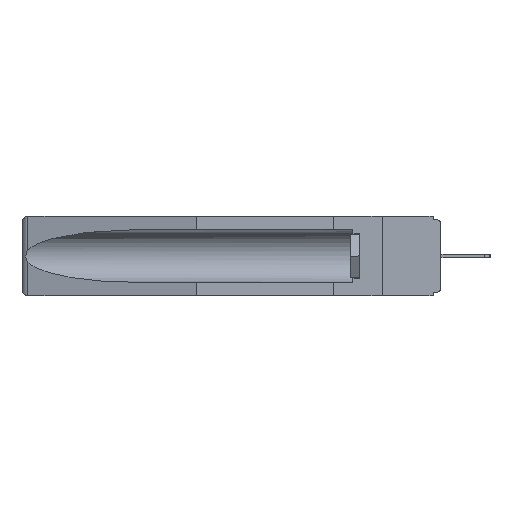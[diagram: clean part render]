
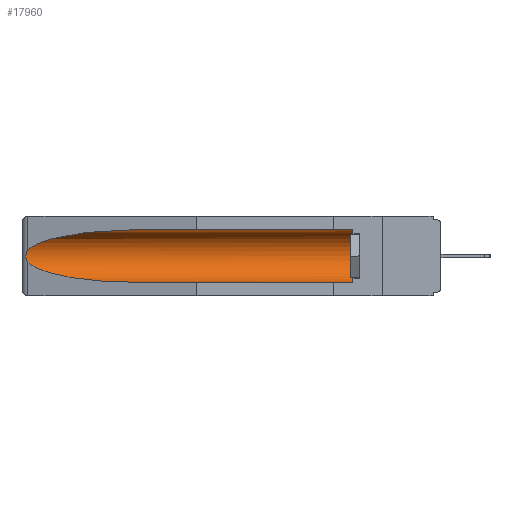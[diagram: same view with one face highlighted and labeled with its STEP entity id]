
A CAD part, left-side view. The second image highlights one B-rep face of the part: STEP entity #17960.
In plain terms, the highlighted cylindrical face has radius 2.857 mm (diameter 5.715 mm), a partial arc.
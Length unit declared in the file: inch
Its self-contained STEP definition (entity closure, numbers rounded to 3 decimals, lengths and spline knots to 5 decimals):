
#262 = DIRECTION ( 'NONE',  ( 0., 0., 1. ) ) ;
#446 = CARTESIAN_POINT ( 'NONE',  ( 0.155, 1.07973, -0.059 ) ) ;
#783 =( BOUNDED_CURVE ( )  B_SPLINE_CURVE ( 3, ( #446, #19437, #3836, #19194 ),
 .UNSPECIFIED., .F., .F. ) 
 B_SPLINE_CURVE_WITH_KNOTS ( ( 4, 4 ),
 ( 4.71239, 6.08839 ),
 .UNSPECIFIED. ) 
 CURVE ( )  GEOMETRIC_REPRESENTATION_ITEM ( )  RATIONAL_B_SPLINE_CURVE ( ( 1., 0.848, 0.848, 1. ) ) 
 REPRESENTATION_ITEM ( '' )  );
#1286 = DIRECTION ( 'NONE',  ( 0., 1., 0. ) ) ;
#1420 = CYLINDRICAL_SURFACE ( 'NONE', #16851, 0.1125 ) ;
#1552 = CARTESIAN_POINT ( 'NONE',  ( 0.2675, 1.53308, -0.16763 ) ) ;
#2125 = CARTESIAN_POINT ( 'NONE',  ( 0.21114, 1.30732, -0.284 ) ) ;
#3092 = ORIENTED_EDGE ( 'NONE', *, *, #8619, .T. ) ;
#3242 = CARTESIAN_POINT ( 'NONE',  ( 0.26537, 1.52718, -0.14972 ) ) ;
#3561 = VERTEX_POINT ( 'NONE', #3242 ) ;
#3836 = CARTESIAN_POINT ( 'NONE',  ( 0.25451, 1.48313, -0.09465 ) ) ;
#3982 = CARTESIAN_POINT ( 'NONE',  ( 0.155, 1.07973, -0.284 ) ) ;
#3990 = DIRECTION ( 'NONE',  ( 0., -1., 0. ) ) ;
#4270 = CARTESIAN_POINT ( 'NONE',  ( 0.26537, 1.52718, -0.19328 ) ) ;
#6153 = EDGE_CURVE ( 'NONE', #14629, #21802, #11021, .T. ) ;
#7290 = CARTESIAN_POINT ( 'NONE',  ( 0.26655, 1.53094, -0.18657 ) ) ;
#7360 =( BOUNDED_CURVE ( )  B_SPLINE_CURVE ( 3, ( #7500, #21107, #2125, #3982 ),
 .UNSPECIFIED., .F., .F. ) 
 B_SPLINE_CURVE_WITH_KNOTS ( ( 4, 4 ),
 ( 0.1948, 1.5708 ),
 .UNSPECIFIED. ) 
 CURVE ( )  GEOMETRIC_REPRESENTATION_ITEM ( )  RATIONAL_B_SPLINE_CURVE ( ( 1., 0.848, 0.848, 1. ) ) 
 REPRESENTATION_ITEM ( '' )  );
#7500 = CARTESIAN_POINT ( 'NONE',  ( 0.26537, 1.52718, -0.19328 ) ) ;
#7736 = ORIENTED_EDGE ( 'NONE', *, *, #19587, .F. ) ;
#8593 = CARTESIAN_POINT ( 'NONE',  ( 0.155, -0.30754, -0.284 ) ) ;
#8619 = EDGE_CURVE ( 'NONE', #20771, #14629, #17702, .T. ) ;
#9035 = CARTESIAN_POINT ( 'NONE',  ( 0.26654, 1.53092, -0.15636 ) ) ;
#9151 = CARTESIAN_POINT ( 'NONE',  ( 0.2675, 1.53308, -0.17534 ) ) ;
#9390 = DIRECTION ( 'NONE',  ( 0., 1., 0. ) ) ;
#9406 = CARTESIAN_POINT ( 'NONE',  ( 0.26597, 1.52961, -0.15275 ) ) ;
#9712 = VERTEX_POINT ( 'NONE', #18661 ) ;
#10483 = ORIENTED_EDGE ( 'NONE', *, *, #6153, .T. ) ;
#10973 = DIRECTION ( 'NONE',  ( 0., 1., 0. ) ) ;
#11021 = LINE ( 'NONE', #16517, #24428 ) ;
#11032 = CARTESIAN_POINT ( 'NONE',  ( 0.155, -0.30754, -0.1715 ) ) ;
#11049 = CARTESIAN_POINT ( 'NONE',  ( 0.26537, 1.52718, -0.14972 ) ) ;
#11100 = EDGE_CURVE ( 'NONE', #3561, #13712, #11937, .T. ) ;
#11937 = B_SPLINE_CURVE_WITH_KNOTS ( 'NONE', 3,
 ( #11049, #9406, #9035, #18665, #1552, #9151, #24423, #7290, #17286, #23157 ),
 .UNSPECIFIED., .F., .F.,
 ( 4, 2, 2, 2, 4 ),
 ( 0., 0.00029, 0.00058, 0.00087, 0.00117 ),
 .UNSPECIFIED. ) ;
#13273 = DIRECTION ( 'NONE',  ( 0., 0., 1. ) ) ;
#13712 = VERTEX_POINT ( 'NONE', #4270 ) ;
#14629 = VERTEX_POINT ( 'NONE', #16070 ) ;
#16070 = CARTESIAN_POINT ( 'NONE',  ( 0.155, 0.126, -0.059 ) ) ;
#16517 = CARTESIAN_POINT ( 'NONE',  ( 0.155, -0.30754, -0.059 ) ) ;
#16851 = AXIS2_PLACEMENT_3D ( 'NONE', #11032, #9390, #13273 ) ;
#17286 = CARTESIAN_POINT ( 'NONE',  ( 0.26597, 1.5296, -0.19026 ) ) ;
#17380 = CARTESIAN_POINT ( 'NONE',  ( 0.155, 0.126, -0.1715 ) ) ;
#17702 = CIRCLE ( 'NONE', #22910, 0.1125 ) ;
#17960 = ADVANCED_FACE ( 'NONE', ( #20527 ), #1420, .F. ) ;
#17985 = ORIENTED_EDGE ( 'NONE', *, *, #18887, .T. ) ;
#18224 = LINE ( 'NONE', #8593, #20502 ) ;
#18339 = CARTESIAN_POINT ( 'NONE',  ( 0.155, 1.07973, -0.059 ) ) ;
#18661 = CARTESIAN_POINT ( 'NONE',  ( 0.155, 1.07973, -0.284 ) ) ;
#18665 = CARTESIAN_POINT ( 'NONE',  ( 0.2673, 1.5327, -0.16383 ) ) ;
#18743 = ORIENTED_EDGE ( 'NONE', *, *, #11100, .T. ) ;
#18887 = EDGE_CURVE ( 'NONE', #21802, #3561, #783, .T. ) ;
#19194 = CARTESIAN_POINT ( 'NONE',  ( 0.26537, 1.52718, -0.14972 ) ) ;
#19240 = EDGE_CURVE ( 'NONE', #13712, #9712, #7360, .T. ) ;
#19437 = CARTESIAN_POINT ( 'NONE',  ( 0.21114, 1.30732, -0.059 ) ) ;
#19587 = EDGE_CURVE ( 'NONE', #20771, #9712, #18224, .T. ) ;
#20502 = VECTOR ( 'NONE', #10973, 39.37008 ) ;
#20527 = FACE_OUTER_BOUND ( 'NONE', #22983, .T. ) ;
#20771 = VERTEX_POINT ( 'NONE', #22475 ) ;
#21107 = CARTESIAN_POINT ( 'NONE',  ( 0.25451, 1.48313, -0.24835 ) ) ;
#21802 = VERTEX_POINT ( 'NONE', #18339 ) ;
#22475 = CARTESIAN_POINT ( 'NONE',  ( 0.155, 0.126, -0.284 ) ) ;
#22832 = ORIENTED_EDGE ( 'NONE', *, *, #19240, .T. ) ;
#22910 = AXIS2_PLACEMENT_3D ( 'NONE', #17380, #3990, #262 ) ;
#22983 = EDGE_LOOP ( 'NONE', ( #17985, #18743, #22832, #7736, #3092, #10483 ) ) ;
#23157 = CARTESIAN_POINT ( 'NONE',  ( 0.26537, 1.52718, -0.19328 ) ) ;
#24423 = CARTESIAN_POINT ( 'NONE',  ( 0.2673, 1.53269, -0.17917 ) ) ;
#24428 = VECTOR ( 'NONE', #1286, 39.37008 ) ;
